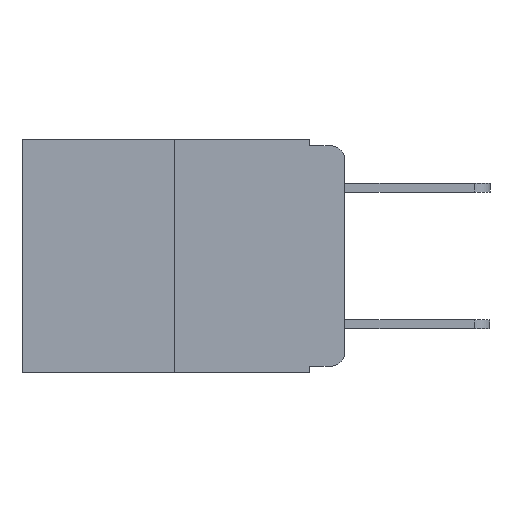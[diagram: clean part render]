
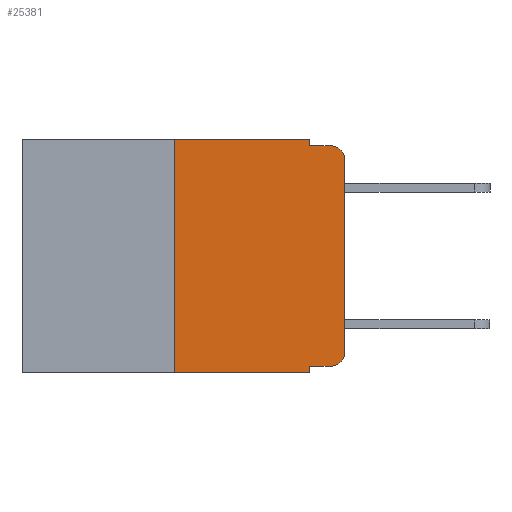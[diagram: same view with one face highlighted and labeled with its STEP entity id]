
A CAD part, left-side view. The second image highlights one B-rep face of the part: STEP entity #25381.
In plain terms, the highlighted planar face has unit normal (-1, 0, 0).
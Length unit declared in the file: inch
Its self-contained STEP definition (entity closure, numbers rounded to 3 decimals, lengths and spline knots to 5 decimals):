
#150 = LINE ( 'NONE', #1367, #10276 ) ;
#572 = VERTEX_POINT ( 'NONE', #4368 ) ;
#1367 = CARTESIAN_POINT ( 'NONE',  ( 0., 0.051, 0. ) ) ;
#1460 = DIRECTION ( 'NONE',  ( 0., 0., -1. ) ) ;
#1589 = LINE ( 'NONE', #9120, #17505 ) ;
#2183 = CARTESIAN_POINT ( 'NONE',  ( 0., 0., -0.03 ) ) ;
#2333 = ORIENTED_EDGE ( 'NONE', *, *, #8836, .F. ) ;
#2632 = ORIENTED_EDGE ( 'NONE', *, *, #16505, .T. ) ;
#3062 = VERTEX_POINT ( 'NONE', #25739 ) ;
#3551 = EDGE_CURVE ( 'NONE', #18137, #16139, #20936, .T. ) ;
#3610 = ORIENTED_EDGE ( 'NONE', *, *, #19514, .F. ) ;
#3911 = ORIENTED_EDGE ( 'NONE', *, *, #8363, .T. ) ;
#4368 = CARTESIAN_POINT ( 'NONE',  ( 0., 0.051, 0. ) ) ;
#4477 = FACE_OUTER_BOUND ( 'NONE', #13636, .T. ) ;
#5094 = VECTOR ( 'NONE', #23457, 39.37008 ) ;
#5763 = CARTESIAN_POINT ( 'NONE',  ( 0., 0.25, -0.343 ) ) ;
#5924 = VECTOR ( 'NONE', #25446, 39.37008 ) ;
#6690 = ORIENTED_EDGE ( 'NONE', *, *, #23145, .F. ) ;
#6789 = DIRECTION ( 'NONE',  ( 0., 0., -1. ) ) ;
#6944 = VECTOR ( 'NONE', #22828, 39.37008 ) ;
#7297 = VERTEX_POINT ( 'NONE', #25847 ) ;
#7612 = ORIENTED_EDGE ( 'NONE', *, *, #12394, .T. ) ;
#7970 = DIRECTION ( 'NONE',  ( -1., 0., 0. ) ) ;
#8363 = EDGE_CURVE ( 'NONE', #8437, #25549, #23404, .T. ) ;
#8437 = VERTEX_POINT ( 'NONE', #2183 ) ;
#8836 = EDGE_CURVE ( 'NONE', #16139, #572, #18742, .T. ) ;
#8928 = LINE ( 'NONE', #24839, #9575 ) ;
#9120 = CARTESIAN_POINT ( 'NONE',  ( 0., 0.051, -0.333 ) ) ;
#9231 = DIRECTION ( 'NONE',  ( -1., 0., 0. ) ) ;
#9575 = VECTOR ( 'NONE', #11055, 39.37008 ) ;
#9621 = CARTESIAN_POINT ( 'NONE',  ( 0., 0.25, 0. ) ) ;
#9724 = VERTEX_POINT ( 'NONE', #21849 ) ;
#10033 = CARTESIAN_POINT ( 'NONE',  ( 0., 0., 0. ) ) ;
#10133 = CARTESIAN_POINT ( 'NONE',  ( 0., 0.051, -0.01 ) ) ;
#10276 = VECTOR ( 'NONE', #1460, 39.37008 ) ;
#10332 = AXIS2_PLACEMENT_3D ( 'NONE', #21113, #9231, #23084 ) ;
#10590 = VECTOR ( 'NONE', #22055, 39.37008 ) ;
#11055 = DIRECTION ( 'NONE',  ( 0., 0., -1. ) ) ;
#11663 = VERTEX_POINT ( 'NONE', #18281 ) ;
#11674 = CARTESIAN_POINT ( 'NONE',  ( 0., 0.473, -0.343 ) ) ;
#11872 = LINE ( 'NONE', #11674, #5924 ) ;
#11955 = CIRCLE ( 'NONE', #10332, 0.02 ) ;
#12394 = EDGE_CURVE ( 'NONE', #9724, #8437, #21140, .T. ) ;
#13636 = EDGE_LOOP ( 'NONE', ( #7612, #3911, #3610, #16984, #2333, #25320, #15406, #6690, #2632, #18824 ) ) ;
#13842 = CARTESIAN_POINT ( 'NONE',  ( 0., 0.25, 0. ) ) ;
#14115 = DIRECTION ( 'NONE',  ( 0., -1., 0. ) ) ;
#15406 = ORIENTED_EDGE ( 'NONE', *, *, #18725, .T. ) ;
#15525 = VECTOR ( 'NONE', #14115, 39.37008 ) ;
#15703 = VERTEX_POINT ( 'NONE', #22414 ) ;
#16139 = VERTEX_POINT ( 'NONE', #13842 ) ;
#16505 = EDGE_CURVE ( 'NONE', #11663, #7297, #1589, .T. ) ;
#16681 = PLANE ( 'NONE',  #24066 ) ;
#16984 = ORIENTED_EDGE ( 'NONE', *, *, #21344, .F. ) ;
#17111 = CARTESIAN_POINT ( 'NONE',  ( 0., 0.02, -0.01 ) ) ;
#17505 = VECTOR ( 'NONE', #21008, 39.37008 ) ;
#18137 = VERTEX_POINT ( 'NONE', #5763 ) ;
#18281 = CARTESIAN_POINT ( 'NONE',  ( 0., 0.051, -0.333 ) ) ;
#18668 = DIRECTION ( 'NONE',  ( 1., 0., 0. ) ) ;
#18725 = EDGE_CURVE ( 'NONE', #18137, #15703, #11872, .T. ) ;
#18742 = LINE ( 'NONE', #24705, #6944 ) ;
#18824 = ORIENTED_EDGE ( 'NONE', *, *, #25516, .T. ) ;
#19514 = EDGE_CURVE ( 'NONE', #3062, #25549, #24775, .T. ) ;
#19851 = CARTESIAN_POINT ( 'NONE',  ( 0., 0.02, -0.03 ) ) ;
#20936 = LINE ( 'NONE', #9621, #5094 ) ;
#21008 = DIRECTION ( 'NONE',  ( 0., -1., 0. ) ) ;
#21113 = CARTESIAN_POINT ( 'NONE',  ( 0., 0.02, -0.313 ) ) ;
#21140 = LINE ( 'NONE', #10033, #10590 ) ;
#21344 = EDGE_CURVE ( 'NONE', #572, #3062, #150, .T. ) ;
#21849 = CARTESIAN_POINT ( 'NONE',  ( 0., 0., -0.313 ) ) ;
#21856 = DIRECTION ( 'NONE',  ( 0., 0., -1. ) ) ;
#22055 = DIRECTION ( 'NONE',  ( 0., 0., 1. ) ) ;
#22414 = CARTESIAN_POINT ( 'NONE',  ( 0., 0.051, -0.343 ) ) ;
#22828 = DIRECTION ( 'NONE',  ( 0., -1., 0. ) ) ;
#23084 = DIRECTION ( 'NONE',  ( 0., 0., -1. ) ) ;
#23145 = EDGE_CURVE ( 'NONE', #11663, #15703, #8928, .T. ) ;
#23404 = CIRCLE ( 'NONE', #23957, 0.02 ) ;
#23457 = DIRECTION ( 'NONE',  ( 0., 0., 1. ) ) ;
#23957 = AXIS2_PLACEMENT_3D ( 'NONE', #19851, #7970, #21856 ) ;
#24066 = AXIS2_PLACEMENT_3D ( 'NONE', #24528, #18668, #6789 ) ;
#24528 = CARTESIAN_POINT ( 'NONE',  ( 0., 0.473, 0. ) ) ;
#24705 = CARTESIAN_POINT ( 'NONE',  ( 0., 0.473, 0. ) ) ;
#24775 = LINE ( 'NONE', #10133, #15525 ) ;
#24839 = CARTESIAN_POINT ( 'NONE',  ( 0., 0.051, 0. ) ) ;
#25320 = ORIENTED_EDGE ( 'NONE', *, *, #3551, .F. ) ;
#25381 = ADVANCED_FACE ( 'NONE', ( #4477 ), #16681, .F. ) ;
#25446 = DIRECTION ( 'NONE',  ( 0., -1., 0. ) ) ;
#25516 = EDGE_CURVE ( 'NONE', #7297, #9724, #11955, .T. ) ;
#25549 = VERTEX_POINT ( 'NONE', #17111 ) ;
#25739 = CARTESIAN_POINT ( 'NONE',  ( 0., 0.051, -0.01 ) ) ;
#25847 = CARTESIAN_POINT ( 'NONE',  ( 0., 0.02, -0.333 ) ) ;
